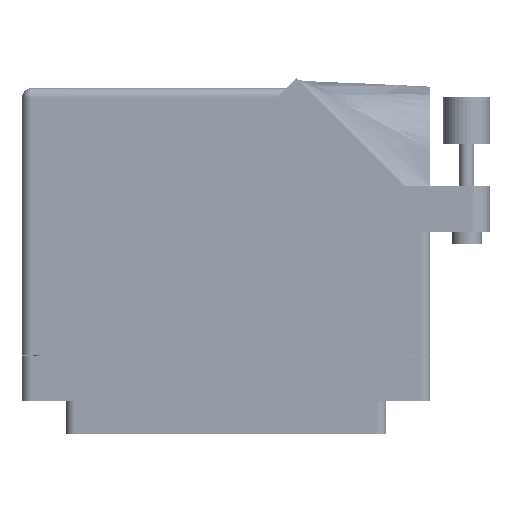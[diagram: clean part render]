
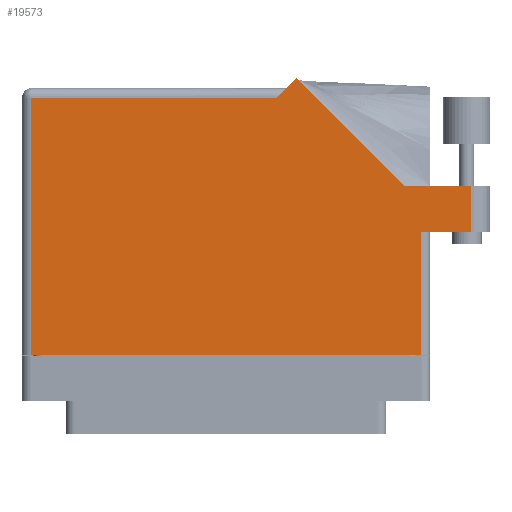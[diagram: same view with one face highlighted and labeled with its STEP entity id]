
A CAD part, front view. The second image highlights one B-rep face of the part: STEP entity #19573.
In plain terms, the highlighted face is planar.
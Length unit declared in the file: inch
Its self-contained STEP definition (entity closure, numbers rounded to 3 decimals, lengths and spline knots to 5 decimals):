
#644 = CARTESIAN_POINT ( 'NONE',  ( 1.634, 1.022, 0.617 ) ) ;
#1488 = ORIENTED_EDGE ( 'NONE', *, *, #6105, .T. ) ;
#1786 = VECTOR ( 'NONE', #22802, 39.37008 ) ;
#2634 = LINE ( 'NONE', #21950, #31193 ) ;
#4577 = DIRECTION ( 'NONE',  ( -0.707, 0.707, 0. ) ) ;
#5833 = VERTEX_POINT ( 'NONE', #25446 ) ;
#6105 = EDGE_CURVE ( 'NONE', #5833, #16917, #71358, .T. ) ;
#7920 = LINE ( 'NONE', #47114, #41870 ) ;
#8075 = FACE_OUTER_BOUND ( 'NONE', #57419, .T. ) ;
#8838 = ORIENTED_EDGE ( 'NONE', *, *, #66434, .T. ) ;
#8877 = ORIENTED_EDGE ( 'NONE', *, *, #11709, .T. ) ;
#10672 = ORIENTED_EDGE ( 'NONE', *, *, #37379, .T. ) ;
#10733 = DIRECTION ( 'NONE',  ( 1., 0., 0. ) ) ;
#11210 = EDGE_CURVE ( 'NONE', #49575, #15739, #2634, .T. ) ;
#11575 = DIRECTION ( 'NONE',  ( -1., 0., 0. ) ) ;
#11709 = EDGE_CURVE ( 'NONE', #21819, #49575, #7920, .T. ) ;
#12157 = DIRECTION ( 'NONE',  ( 0., 1., 0. ) ) ;
#12865 = EDGE_CURVE ( 'NONE', #16917, #48117, #30100, .T. ) ;
#13723 = CARTESIAN_POINT ( 'NONE',  ( 0.46971, 1.74571, 0.617 ) ) ;
#14792 = DIRECTION ( 'NONE',  ( -1., 0., 0. ) ) ;
#15739 = VERTEX_POINT ( 'NONE', #27531 ) ;
#16692 = EDGE_CURVE ( 'NONE', #15739, #5833, #48278, .T. ) ;
#16917 = VERTEX_POINT ( 'NONE', #25575 ) ;
#17042 = LINE ( 'NONE', #73864, #30352 ) ;
#17837 = VECTOR ( 'NONE', #34350, 39.37008 ) ;
#19573 = ADVANCED_FACE ( 'NONE', ( #8075 ), #60855, .F. ) ;
#21819 = VERTEX_POINT ( 'NONE', #57876 ) ;
#21950 = CARTESIAN_POINT ( 'NONE',  ( 1.359, 0.715, 0.617 ) ) ;
#22048 = VERTEX_POINT ( 'NONE', #60842 ) ;
#22802 = DIRECTION ( 'NONE',  ( -1., 0., 0. ) ) ;
#25175 = DIRECTION ( 'NONE',  ( 1., 0., 0. ) ) ;
#25446 = CARTESIAN_POINT ( 'NONE',  ( 1.634, 1.022, 0.617 ) ) ;
#25575 = CARTESIAN_POINT ( 'NONE',  ( 1.19342, 1.022, 0.617 ) ) ;
#26209 = CARTESIAN_POINT ( 'NONE',  ( 0.337, 1.613, 0.617 ) ) ;
#26555 = VECTOR ( 'NONE', #25175, 39.37008 ) ;
#27531 = CARTESIAN_POINT ( 'NONE',  ( 1.634, 0.715, 0.617 ) ) ;
#28825 = ORIENTED_EDGE ( 'NONE', *, *, #34673, .T. ) ;
#30100 = LINE ( 'NONE', #30426, #34549 ) ;
#30352 = VECTOR ( 'NONE', #11575, 39.37008 ) ;
#30426 = CARTESIAN_POINT ( 'NONE',  ( 1.19342, 1.022, 0.617 ) ) ;
#31193 = VECTOR ( 'NONE', #10733, 39.37008 ) ;
#32947 = LINE ( 'NONE', #51768, #17837 ) ;
#34350 = DIRECTION ( 'NONE',  ( 0., -1., 0. ) ) ;
#34541 = ORIENTED_EDGE ( 'NONE', *, *, #16692, .T. ) ;
#34549 = VECTOR ( 'NONE', #4577, 39.37008 ) ;
#34673 = EDGE_CURVE ( 'NONE', #22048, #21819, #64872, .T. ) ;
#36578 = VERTEX_POINT ( 'NONE', #66416 ) ;
#37379 = EDGE_CURVE ( 'NONE', #48117, #67999, #44072, .T. ) ;
#38300 = CARTESIAN_POINT ( 'NONE',  ( 1.297, 0.715, 0.617 ) ) ;
#39537 = DIRECTION ( 'NONE',  ( -0.707, -0.707, 0. ) ) ;
#41870 = VECTOR ( 'NONE', #46862, 39.37008 ) ;
#44072 = LINE ( 'NONE', #61246, #60191 ) ;
#46862 = DIRECTION ( 'NONE',  ( 0., 1., 0. ) ) ;
#47114 = CARTESIAN_POINT ( 'NONE',  ( 1.297, 0.715, 0.617 ) ) ;
#48117 = VERTEX_POINT ( 'NONE', #13723 ) ;
#48278 = LINE ( 'NONE', #644, #72391 ) ;
#48444 = AXIS2_PLACEMENT_3D ( 'NONE', #66092, #60383, #14792 ) ;
#49575 = VERTEX_POINT ( 'NONE', #38300 ) ;
#50292 = EDGE_CURVE ( 'NONE', #36578, #22048, #32947, .T. ) ;
#51768 = CARTESIAN_POINT ( 'NONE',  ( -1.297, -0.1, 0.617 ) ) ;
#56719 = ORIENTED_EDGE ( 'NONE', *, *, #11210, .T. ) ;
#57419 = EDGE_LOOP ( 'NONE', ( #56719, #34541, #1488, #72726, #10672, #8838, #73873, #28825, #8877 ) ) ;
#57876 = CARTESIAN_POINT ( 'NONE',  ( 1.297, -0.1, 0.617 ) ) ;
#59294 = CARTESIAN_POINT ( 'NONE',  ( -1.359, -0.1, 0.617 ) ) ;
#60191 = VECTOR ( 'NONE', #39537, 39.37008 ) ;
#60383 = DIRECTION ( 'NONE',  ( 0., 0., -1. ) ) ;
#60842 = CARTESIAN_POINT ( 'NONE',  ( -1.297, -0.1, 0.617 ) ) ;
#60855 = PLANE ( 'NONE',  #48444 ) ;
#61246 = CARTESIAN_POINT ( 'NONE',  ( 0.399, 1.675, 0.617 ) ) ;
#64872 = LINE ( 'NONE', #59294, #26555 ) ;
#65700 = CARTESIAN_POINT ( 'NONE',  ( 1.759, 1.022, 0.617 ) ) ;
#66092 = CARTESIAN_POINT ( 'NONE',  ( -1.359, 1.675, 0.617 ) ) ;
#66416 = CARTESIAN_POINT ( 'NONE',  ( -1.297, 1.613, 0.617 ) ) ;
#66434 = EDGE_CURVE ( 'NONE', #67999, #36578, #17042, .T. ) ;
#67999 = VERTEX_POINT ( 'NONE', #26209 ) ;
#71358 = LINE ( 'NONE', #65700, #1786 ) ;
#72391 = VECTOR ( 'NONE', #12157, 39.37008 ) ;
#72726 = ORIENTED_EDGE ( 'NONE', *, *, #12865, .T. ) ;
#73864 = CARTESIAN_POINT ( 'NONE',  ( -1.359, 1.613, 0.617 ) ) ;
#73873 = ORIENTED_EDGE ( 'NONE', *, *, #50292, .T. ) ;
